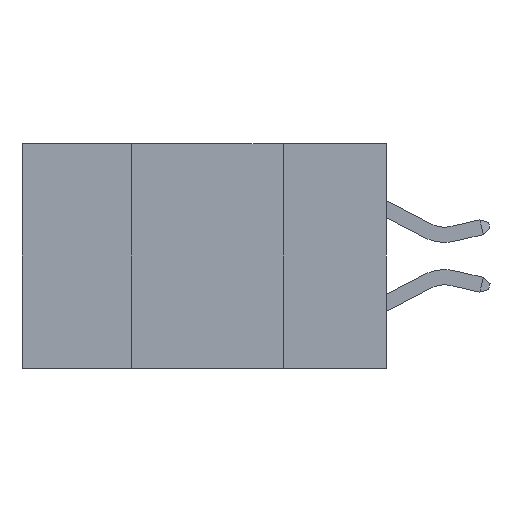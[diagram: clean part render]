
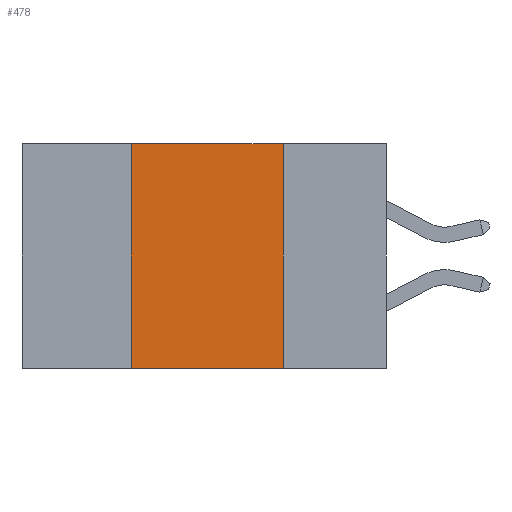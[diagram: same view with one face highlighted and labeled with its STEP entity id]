
A CAD part, left-side view. The second image highlights one B-rep face of the part: STEP entity #478.
In plain terms, the highlighted planar face has unit normal (-1, 0, 0).
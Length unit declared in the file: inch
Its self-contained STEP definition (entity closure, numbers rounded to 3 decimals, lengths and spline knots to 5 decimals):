
#478 = ADVANCED_FACE ( 'NONE', ( #23653 ), #21931, .F. ) ;
#1518 = CARTESIAN_POINT ( 'NONE',  ( 0., 0.17, 0. ) ) ;
#2565 = VERTEX_POINT ( 'NONE', #28139 ) ;
#2654 = CARTESIAN_POINT ( 'NONE',  ( 0., 0.42, 0. ) ) ;
#4099 = VECTOR ( 'NONE', #14840, 39.37008 ) ;
#5492 = EDGE_CURVE ( 'NONE', #28092, #2565, #13815, .T. ) ;
#7111 = ORIENTED_EDGE ( 'NONE', *, *, #23172, .F. ) ;
#7836 = CARTESIAN_POINT ( 'NONE',  ( 0., 0.17, 0. ) ) ;
#8243 = VECTOR ( 'NONE', #20826, 39.37008 ) ;
#8602 = ORIENTED_EDGE ( 'NONE', *, *, #17299, .F. ) ;
#9011 = LINE ( 'NONE', #18722, #8243 ) ;
#9091 = VECTOR ( 'NONE', #31498, 39.37008 ) ;
#10584 = VECTOR ( 'NONE', #15417, 39.37008 ) ;
#13815 = LINE ( 'NONE', #1518, #9091 ) ;
#14840 = DIRECTION ( 'NONE',  ( 0., 0., 1. ) ) ;
#15417 = DIRECTION ( 'NONE',  ( 0., -1., 0. ) ) ;
#16671 = ORIENTED_EDGE ( 'NONE', *, *, #5492, .F. ) ;
#16715 = CARTESIAN_POINT ( 'NONE',  ( 0., 0.42, 0. ) ) ;
#17114 = DIRECTION ( 'NONE',  ( 1., 0., 0. ) ) ;
#17299 = EDGE_CURVE ( 'NONE', #29437, #31493, #31425, .T. ) ;
#17331 = DIRECTION ( 'NONE',  ( 0., 0., -1. ) ) ;
#18722 = CARTESIAN_POINT ( 'NONE',  ( 0., 0.6, 0. ) ) ;
#19228 = EDGE_LOOP ( 'NONE', ( #16671, #7111, #8602, #19374 ) ) ;
#19374 = ORIENTED_EDGE ( 'NONE', *, *, #22860, .T. ) ;
#20211 = CARTESIAN_POINT ( 'NONE',  ( 0., 0.6, -0.37 ) ) ;
#20826 = DIRECTION ( 'NONE',  ( 0., -1., 0. ) ) ;
#21931 = PLANE ( 'NONE',  #25188 ) ;
#22045 = CARTESIAN_POINT ( 'NONE',  ( 0., 0.6, 0. ) ) ;
#22860 = EDGE_CURVE ( 'NONE', #29437, #2565, #30146, .T. ) ;
#23172 = EDGE_CURVE ( 'NONE', #31493, #28092, #9011, .T. ) ;
#23653 = FACE_OUTER_BOUND ( 'NONE', #19228, .T. ) ;
#25188 = AXIS2_PLACEMENT_3D ( 'NONE', #22045, #17114, #17331 ) ;
#27906 = CARTESIAN_POINT ( 'NONE',  ( 0., 0.42, -0.37 ) ) ;
#28092 = VERTEX_POINT ( 'NONE', #7836 ) ;
#28139 = CARTESIAN_POINT ( 'NONE',  ( 0., 0.17, -0.37 ) ) ;
#29437 = VERTEX_POINT ( 'NONE', #27906 ) ;
#30146 = LINE ( 'NONE', #20211, #10584 ) ;
#31425 = LINE ( 'NONE', #2654, #4099 ) ;
#31493 = VERTEX_POINT ( 'NONE', #16715 ) ;
#31498 = DIRECTION ( 'NONE',  ( 0., 0., -1. ) ) ;
